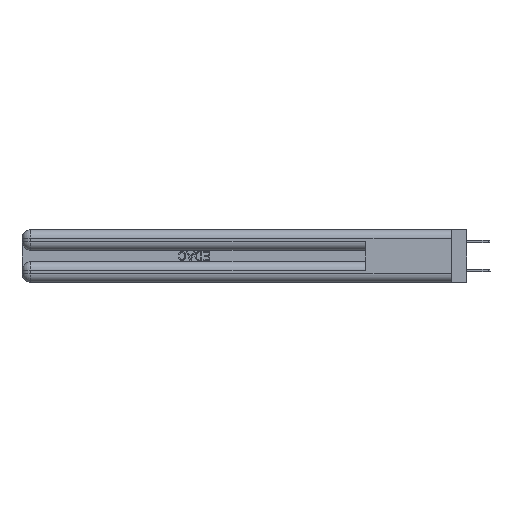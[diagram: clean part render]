
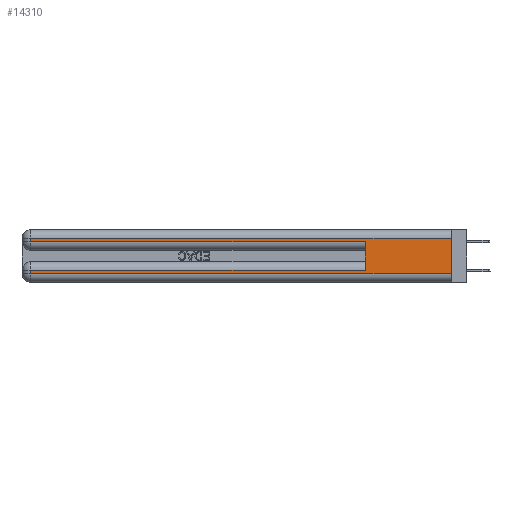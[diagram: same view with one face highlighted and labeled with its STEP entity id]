
A CAD part, left-side view. The second image highlights one B-rep face of the part: STEP entity #14310.
In plain terms, the highlighted planar face has unit normal (-1, 0, 0).
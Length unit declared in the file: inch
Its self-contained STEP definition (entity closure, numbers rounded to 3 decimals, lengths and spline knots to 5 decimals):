
#266 = CARTESIAN_POINT ( 'NONE',  ( 0., 0., 0.06 ) ) ;
#1148 = EDGE_CURVE ( 'NONE', #43894, #48225, #25606, .T. ) ;
#2080 = ORIENTED_EDGE ( 'NONE', *, *, #25625, .T. ) ;
#2107 = PLANE ( 'NONE',  #15792 ) ;
#2141 = VERTEX_POINT ( 'NONE', #41382 ) ;
#3492 = FACE_OUTER_BOUND ( 'NONE', #47448, .T. ) ;
#4038 = CARTESIAN_POINT ( 'NONE',  ( 0., 0., 0.085 ) ) ;
#4382 = EDGE_CURVE ( 'NONE', #38980, #21060, #23413, .T. ) ;
#4819 = CARTESIAN_POINT ( 'NONE',  ( 0., 2.94, 0.285 ) ) ;
#5440 = CARTESIAN_POINT ( 'NONE',  ( 0., 0., 0.31 ) ) ;
#5978 = CARTESIAN_POINT ( 'NONE',  ( 0., 0., 0.06 ) ) ;
#6125 = LINE ( 'NONE', #12148, #36871 ) ;
#6319 = DIRECTION ( 'NONE',  ( 1., 0., 0. ) ) ;
#7354 = LINE ( 'NONE', #28128, #27453 ) ;
#8504 = CARTESIAN_POINT ( 'NONE',  ( 0., 0., 0.37 ) ) ;
#11129 = CARTESIAN_POINT ( 'NONE',  ( 0., 2.94, 0.085 ) ) ;
#11958 = ORIENTED_EDGE ( 'NONE', *, *, #23143, .F. ) ;
#12148 = CARTESIAN_POINT ( 'NONE',  ( 0., 2.94, 0.37 ) ) ;
#14248 = EDGE_CURVE ( 'NONE', #45405, #18087, #38070, .T. ) ;
#14310 = ADVANCED_FACE ( 'NONE', ( #3492 ), #2107, .F. ) ;
#14939 = VECTOR ( 'NONE', #46574, 39.37008 ) ;
#15484 = VECTOR ( 'NONE', #44670, 39.37008 ) ;
#15792 = AXIS2_PLACEMENT_3D ( 'NONE', #30375, #6319, #34414 ) ;
#15841 = LINE ( 'NONE', #5440, #38440 ) ;
#15842 = ORIENTED_EDGE ( 'NONE', *, *, #31564, .T. ) ;
#16224 = DIRECTION ( 'NONE',  ( 0., 0., -1. ) ) ;
#17697 = EDGE_CURVE ( 'NONE', #38980, #47048, #17730, .T. ) ;
#17730 = LINE ( 'NONE', #4038, #47219 ) ;
#18087 = VERTEX_POINT ( 'NONE', #266 ) ;
#19552 = ORIENTED_EDGE ( 'NONE', *, *, #4382, .F. ) ;
#19907 = CARTESIAN_POINT ( 'NONE',  ( 0., 0.6, 0.145 ) ) ;
#21060 = VERTEX_POINT ( 'NONE', #31336 ) ;
#23143 = EDGE_CURVE ( 'NONE', #2141, #18087, #36805, .T. ) ;
#23413 = LINE ( 'NONE', #19907, #32840 ) ;
#25606 = LINE ( 'NONE', #50424, #14939 ) ;
#25625 = EDGE_CURVE ( 'NONE', #2141, #43894, #15841, .T. ) ;
#26187 = ORIENTED_EDGE ( 'NONE', *, *, #14248, .T. ) ;
#27453 = VECTOR ( 'NONE', #36182, 39.37008 ) ;
#28128 = CARTESIAN_POINT ( 'NONE',  ( 0., 0., 0.285 ) ) ;
#28631 = VECTOR ( 'NONE', #34064, 39.37008 ) ;
#28845 = ORIENTED_EDGE ( 'NONE', *, *, #17697, .T. ) ;
#29459 = ORIENTED_EDGE ( 'NONE', *, *, #31559, .T. ) ;
#29507 = DIRECTION ( 'NONE',  ( 0., 1., 0. ) ) ;
#30014 = ORIENTED_EDGE ( 'NONE', *, *, #1148, .T. ) ;
#30375 = CARTESIAN_POINT ( 'NONE',  ( 0., 0., 0.37 ) ) ;
#31336 = CARTESIAN_POINT ( 'NONE',  ( 0., 0.6, 0.285 ) ) ;
#31559 = EDGE_CURVE ( 'NONE', #48225, #21060, #7354, .T. ) ;
#31564 = EDGE_CURVE ( 'NONE', #47048, #45405, #6125, .T. ) ;
#32840 = VECTOR ( 'NONE', #43923, 39.37008 ) ;
#34064 = DIRECTION ( 'NONE',  ( 0., -1., 0. ) ) ;
#34414 = DIRECTION ( 'NONE',  ( 0., 0., -1. ) ) ;
#36182 = DIRECTION ( 'NONE',  ( 0., -1., 0. ) ) ;
#36805 = LINE ( 'NONE', #8504, #15484 ) ;
#36871 = VECTOR ( 'NONE', #16224, 39.37008 ) ;
#38070 = LINE ( 'NONE', #5978, #28631 ) ;
#38440 = VECTOR ( 'NONE', #29507, 39.37008 ) ;
#38980 = VERTEX_POINT ( 'NONE', #49644 ) ;
#41382 = CARTESIAN_POINT ( 'NONE',  ( 0., 0., 0.31 ) ) ;
#43894 = VERTEX_POINT ( 'NONE', #47735 ) ;
#43923 = DIRECTION ( 'NONE',  ( 0., 0., 1. ) ) ;
#44087 = DIRECTION ( 'NONE',  ( 0., 1., 0. ) ) ;
#44670 = DIRECTION ( 'NONE',  ( 0., 0., -1. ) ) ;
#45184 = CARTESIAN_POINT ( 'NONE',  ( 0., 2.94, 0.06 ) ) ;
#45405 = VERTEX_POINT ( 'NONE', #45184 ) ;
#46574 = DIRECTION ( 'NONE',  ( 0., 0., -1. ) ) ;
#47048 = VERTEX_POINT ( 'NONE', #11129 ) ;
#47219 = VECTOR ( 'NONE', #44087, 39.37008 ) ;
#47448 = EDGE_LOOP ( 'NONE', ( #11958, #2080, #30014, #29459, #19552, #28845, #15842, #26187 ) ) ;
#47735 = CARTESIAN_POINT ( 'NONE',  ( 0., 2.94, 0.31 ) ) ;
#48225 = VERTEX_POINT ( 'NONE', #4819 ) ;
#49644 = CARTESIAN_POINT ( 'NONE',  ( 0., 0.6, 0.085 ) ) ;
#50424 = CARTESIAN_POINT ( 'NONE',  ( 0., 2.94, 0.37 ) ) ;
